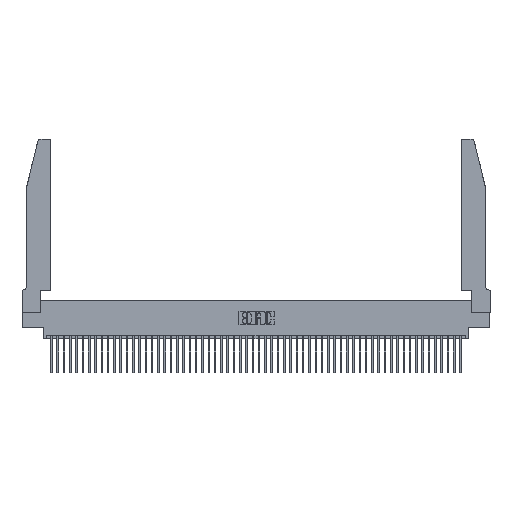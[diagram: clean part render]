
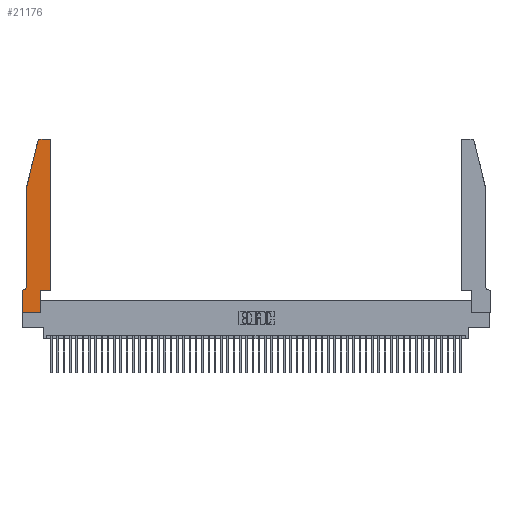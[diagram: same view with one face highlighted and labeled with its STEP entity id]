
A CAD part, top view. The second image highlights one B-rep face of the part: STEP entity #21176.
In plain terms, the highlighted planar face has unit normal (0, 0, 1).
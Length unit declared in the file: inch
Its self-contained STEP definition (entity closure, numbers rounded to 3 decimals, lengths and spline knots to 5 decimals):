
#102 = ORIENTED_EDGE ( 'NONE', *, *, #31868, .T. ) ;
#181 = CARTESIAN_POINT ( 'NONE',  ( 0.25487, 2.72718, 0.37 ) ) ;
#405 = DIRECTION ( 'NONE',  ( 0., 0., 1. ) ) ;
#873 = ORIENTED_EDGE ( 'NONE', *, *, #25458, .T. ) ;
#1093 = CARTESIAN_POINT ( 'NONE',  ( 0.4505, 0.35, 0.37 ) ) ;
#1695 = VECTOR ( 'NONE', #23010, 39.37008 ) ;
#1703 = AXIS2_PLACEMENT_3D ( 'NONE', #26936, #1964, #31047 ) ;
#1964 = DIRECTION ( 'NONE',  ( 0., 0., -1. ) ) ;
#3394 = LINE ( 'NONE', #27715, #14579 ) ;
#4266 = EDGE_CURVE ( 'NONE', #15769, #21223, #3394, .T. ) ;
#4300 = CARTESIAN_POINT ( 'NONE',  ( 0.0755, 2., 0.37 ) ) ;
#5768 = ORIENTED_EDGE ( 'NONE', *, *, #9347, .T. ) ;
#6072 = LINE ( 'NONE', #14880, #36564 ) ;
#6140 = EDGE_CURVE ( 'NONE', #20611, #51671, #6072, .T. ) ;
#6151 = VERTEX_POINT ( 'NONE', #51828 ) ;
#6248 = CARTESIAN_POINT ( 'NONE',  ( 0.2605, 2.75, 0.37 ) ) ;
#6661 = VECTOR ( 'NONE', #22409, 39.37008 ) ;
#6818 = ORIENTED_EDGE ( 'NONE', *, *, #4266, .T. ) ;
#7700 = EDGE_CURVE ( 'NONE', #51671, #15769, #33789, .T. ) ;
#7981 = AXIS2_PLACEMENT_3D ( 'NONE', #36790, #45021, #20406 ) ;
#9054 = CARTESIAN_POINT ( 'NONE',  ( 0., 0., 0.37 ) ) ;
#9347 = EDGE_CURVE ( 'NONE', #28549, #43431, #9659, .T. ) ;
#9659 = CIRCLE ( 'NONE', #43462, 0.03 ) ;
#10663 = DIRECTION ( 'NONE',  ( 0., -1., 0. ) ) ;
#11741 = ORIENTED_EDGE ( 'NONE', *, *, #17622, .T. ) ;
#11753 = CARTESIAN_POINT ( 'NONE',  ( 0.2865, 0., 0.37 ) ) ;
#12788 = LINE ( 'NONE', #19880, #34740 ) ;
#14216 = CARTESIAN_POINT ( 'NONE',  ( 0.0055, 0.35, 0.37 ) ) ;
#14579 = VECTOR ( 'NONE', #15410, 39.37008 ) ;
#14835 = CARTESIAN_POINT ( 'NONE',  ( 0.0755, 2., 0.37 ) ) ;
#14880 = CARTESIAN_POINT ( 'NONE',  ( 0., 0., 0.37 ) ) ;
#15410 = DIRECTION ( 'NONE',  ( 0., 1., 0. ) ) ;
#15462 = ORIENTED_EDGE ( 'NONE', *, *, #47347, .T. ) ;
#15769 = VERTEX_POINT ( 'NONE', #11753 ) ;
#15770 = CARTESIAN_POINT ( 'NONE',  ( 0.284, 2.72, 0.37 ) ) ;
#15942 = ORIENTED_EDGE ( 'NONE', *, *, #6140, .T. ) ;
#16202 = EDGE_CURVE ( 'NONE', #21223, #25051, #38405, .T. ) ;
#16252 = PLANE ( 'NONE',  #7981 ) ;
#16531 = VERTEX_POINT ( 'NONE', #20417 ) ;
#17045 = LINE ( 'NONE', #24577, #49793 ) ;
#17622 = EDGE_CURVE ( 'NONE', #16531, #28549, #34826, .T. ) ;
#19502 = VERTEX_POINT ( 'NONE', #14216 ) ;
#19880 = CARTESIAN_POINT ( 'NONE',  ( 0.0755, 2., 0.37 ) ) ;
#19947 = DIRECTION ( 'NONE',  ( 1., 0., 0. ) ) ;
#20103 = ORIENTED_EDGE ( 'NONE', *, *, #50771, .T. ) ;
#20406 = DIRECTION ( 'NONE',  ( 1., 0., 0. ) ) ;
#20417 = CARTESIAN_POINT ( 'NONE',  ( 0.4205, 2.75, 0.37 ) ) ;
#20567 = CARTESIAN_POINT ( 'NONE',  ( 0.2865, 0.35, 0.37 ) ) ;
#20611 = VERTEX_POINT ( 'NONE', #49681 ) ;
#21176 = ADVANCED_FACE ( 'NONE', ( #50404 ), #16252, .T. ) ;
#21223 = VERTEX_POINT ( 'NONE', #20567 ) ;
#22409 = DIRECTION ( 'NONE',  ( 1., 0., 0. ) ) ;
#23010 = DIRECTION ( 'NONE',  ( -1., 0., 0. ) ) ;
#24032 = EDGE_CURVE ( 'NONE', #19502, #20611, #42959, .T. ) ;
#24212 = CIRCLE ( 'NONE', #1703, 0.07 ) ;
#24577 = CARTESIAN_POINT ( 'NONE',  ( 0.4505, 0.35, 0.37 ) ) ;
#25051 = VERTEX_POINT ( 'NONE', #1093 ) ;
#25058 = CARTESIAN_POINT ( 'NONE',  ( 0.0755, 0.42, 0.37 ) ) ;
#25416 = CARTESIAN_POINT ( 'NONE',  ( 0.4205, 2.72, 0.37 ) ) ;
#25458 = EDGE_CURVE ( 'NONE', #25051, #6151, #17045, .T. ) ;
#26936 = CARTESIAN_POINT ( 'NONE',  ( 0.0055, 0.42, 0.37 ) ) ;
#27715 = CARTESIAN_POINT ( 'NONE',  ( 0.2865, 0.35, 0.37 ) ) ;
#28549 = VERTEX_POINT ( 'NONE', #50394 ) ;
#28771 = VERTEX_POINT ( 'NONE', #14835 ) ;
#29538 = DIRECTION ( 'NONE',  ( 1., 0., 0. ) ) ;
#29846 = EDGE_LOOP ( 'NONE', ( #11741, #5768, #20103, #47703, #15462, #32918, #15942, #38814, #6818, #53216, #873, #102 ) ) ;
#29959 = VECTOR ( 'NONE', #46473, 39.37008 ) ;
#30171 = CARTESIAN_POINT ( 'NONE',  ( 0., 0., 0.37 ) ) ;
#31047 = DIRECTION ( 'NONE',  ( -1., 0., 0. ) ) ;
#31868 = EDGE_CURVE ( 'NONE', #6151, #16531, #35855, .T. ) ;
#32709 = CARTESIAN_POINT ( 'NONE',  ( 0.0755, 0.35, 0.37 ) ) ;
#32918 = ORIENTED_EDGE ( 'NONE', *, *, #24032, .T. ) ;
#33789 = LINE ( 'NONE', #30171, #29959 ) ;
#34740 = VECTOR ( 'NONE', #52627, 39.37008 ) ;
#34826 = LINE ( 'NONE', #6248, #1695 ) ;
#35620 = VECTOR ( 'NONE', #41619, 39.37008 ) ;
#35855 = CIRCLE ( 'NONE', #36082, 0.03 ) ;
#36082 = AXIS2_PLACEMENT_3D ( 'NONE', #25416, #405, #29538 ) ;
#36131 = VERTEX_POINT ( 'NONE', #25058 ) ;
#36564 = VECTOR ( 'NONE', #10663, 39.37008 ) ;
#36790 = CARTESIAN_POINT ( 'NONE',  ( 0., 0.35, 0.37 ) ) ;
#36902 = DIRECTION ( 'NONE',  ( -1., 0., 0. ) ) ;
#38405 = LINE ( 'NONE', #51093, #6661 ) ;
#38814 = ORIENTED_EDGE ( 'NONE', *, *, #7700, .T. ) ;
#41619 = DIRECTION ( 'NONE',  ( 0., -1., 0. ) ) ;
#41682 = VECTOR ( 'NONE', #36902, 39.37008 ) ;
#42959 = LINE ( 'NONE', #32709, #41682 ) ;
#43431 = VERTEX_POINT ( 'NONE', #181 ) ;
#43462 = AXIS2_PLACEMENT_3D ( 'NONE', #15770, #44565, #19947 ) ;
#44565 = DIRECTION ( 'NONE',  ( 0., 0., 1. ) ) ;
#45021 = DIRECTION ( 'NONE',  ( 0., 0., 1. ) ) ;
#46473 = DIRECTION ( 'NONE',  ( 1., 0., 0. ) ) ;
#46494 = LINE ( 'NONE', #4300, #35620 ) ;
#47347 = EDGE_CURVE ( 'NONE', #36131, #19502, #24212, .T. ) ;
#47703 = ORIENTED_EDGE ( 'NONE', *, *, #48851, .T. ) ;
#48851 = EDGE_CURVE ( 'NONE', #28771, #36131, #46494, .T. ) ;
#49681 = CARTESIAN_POINT ( 'NONE',  ( 0., 0.35, 0.37 ) ) ;
#49793 = VECTOR ( 'NONE', #53193, 39.37008 ) ;
#50394 = CARTESIAN_POINT ( 'NONE',  ( 0.284, 2.75, 0.37 ) ) ;
#50404 = FACE_OUTER_BOUND ( 'NONE', #29846, .T. ) ;
#50771 = EDGE_CURVE ( 'NONE', #43431, #28771, #12788, .T. ) ;
#51093 = CARTESIAN_POINT ( 'NONE',  ( 0.4505, 0.35, 0.37 ) ) ;
#51671 = VERTEX_POINT ( 'NONE', #9054 ) ;
#51828 = CARTESIAN_POINT ( 'NONE',  ( 0.4505, 2.72, 0.37 ) ) ;
#52627 = DIRECTION ( 'NONE',  ( -0.239, -0.971, 0. ) ) ;
#53193 = DIRECTION ( 'NONE',  ( 0., 1., 0. ) ) ;
#53216 = ORIENTED_EDGE ( 'NONE', *, *, #16202, .T. ) ;
